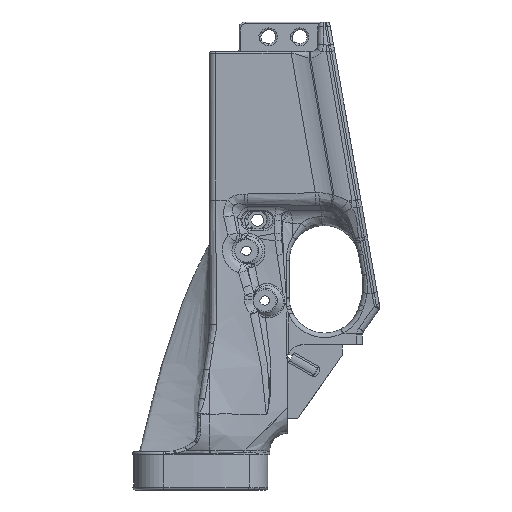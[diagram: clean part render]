
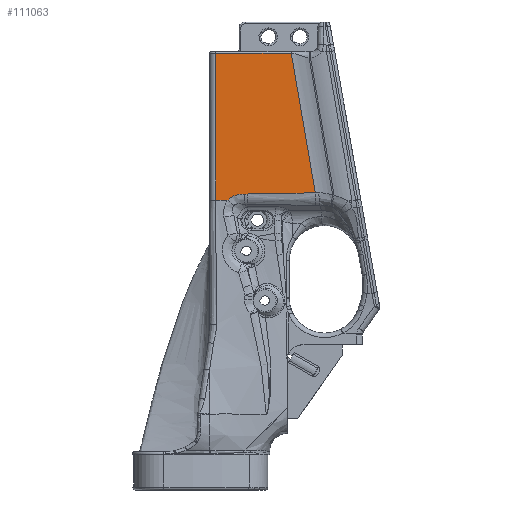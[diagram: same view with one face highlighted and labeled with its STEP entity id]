
A CAD part, left-side view. The second image highlights one B-rep face of the part: STEP entity #111063.
In plain terms, the highlighted planar face has unit normal (-1, 0, 0).
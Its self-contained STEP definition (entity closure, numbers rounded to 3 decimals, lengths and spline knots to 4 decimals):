
#154 = CARTESIAN_POINT ( 'NONE',  ( -0.7, -0.2845, 3.63 ) ) ;
#1696 = EDGE_CURVE ( 'NONE', #95053, #49894, #95486, .T. ) ;
#1853 = CARTESIAN_POINT ( 'NONE',  ( -0.7, -0.2304, 3.63 ) ) ;
#2705 = ORIENTED_EDGE ( 'NONE', *, *, #1696, .T. ) ;
#3995 = CARTESIAN_POINT ( 'NONE',  ( -0.7, -1.7909, 3.7543 ) ) ;
#4014 = DIRECTION ( 'NONE',  ( 0., -1., 0. ) ) ;
#4437 = LINE ( 'NONE', #12462, #68008 ) ;
#8159 = CARTESIAN_POINT ( 'NONE',  ( -0.7, -0.1, 6.12 ) ) ;
#9075 = VECTOR ( 'NONE', #42230, 39.3701 ) ;
#9605 = EDGE_CURVE ( 'NONE', #103485, #88719, #54430, .T. ) ;
#10171 = ORIENTED_EDGE ( 'NONE', *, *, #54507, .F. ) ;
#12462 = CARTESIAN_POINT ( 'NONE',  ( -0.7, 0., 6.12 ) ) ;
#13210 = CARTESIAN_POINT ( 'NONE',  ( -0.7, -0.5916, 3.7336 ) ) ;
#13559 = AXIS2_PLACEMENT_3D ( 'NONE', #17843, #69344, #61894 ) ;
#15915 = CARTESIAN_POINT ( 'NONE',  ( -0.7, -1.4229, 5.8986 ) ) ;
#17333 = EDGE_CURVE ( 'NONE', #108173, #111315, #99951, .T. ) ;
#17843 = CARTESIAN_POINT ( 'NONE',  ( -0.7, -2.8877, 6.15 ) ) ;
#17896 = CARTESIAN_POINT ( 'NONE',  ( -0.7, -0.1, 3.63 ) ) ;
#20760 = EDGE_LOOP ( 'NONE', ( #93236, #26798, #106490, #10171, #74144, #101146, #53672, #2705 ) ) ;
#23035 = CARTESIAN_POINT ( 'NONE',  ( -0.7, -0.4525, 3.7151 ) ) ;
#24162 = CARTESIAN_POINT ( 'NONE',  ( -0.7, -0.3296, 3.6483 ) ) ;
#25581 = CARTESIAN_POINT ( 'NONE',  ( -0.7, -0.3116, 3.63 ) ) ;
#26413 = CARTESIAN_POINT ( 'NONE',  ( -0.7, -0.2304, 3.63 ) ) ;
#26508 = CARTESIAN_POINT ( 'NONE',  ( -0.7, -0.3116, 3.63 ) ) ;
#26798 = ORIENTED_EDGE ( 'NONE', *, *, #48734, .T. ) ;
#28096 = CARTESIAN_POINT ( 'NONE',  ( -0.7, -0.64, 3.7336 ) ) ;
#28221 = CARTESIAN_POINT ( 'NONE',  ( -0.7, -0.1869, 3.63 ) ) ;
#28793 = CARTESIAN_POINT ( 'NONE',  ( -0.7, -0.2304, 3.63 ) ) ;
#29260 = LINE ( 'NONE', #108776, #111168 ) ;
#30536 = CARTESIAN_POINT ( 'NONE',  ( -0.7, -0.3495, 3.6646 ) ) ;
#35581 = FACE_OUTER_BOUND ( 'NONE', #20760, .T. ) ;
#35969 = EDGE_CURVE ( 'NONE', #48324, #95053, #98297, .T. ) ;
#38367 = CARTESIAN_POINT ( 'NONE',  ( -0.7, -1.0236, 3.7336 ) ) ;
#40769 = CARTESIAN_POINT ( 'NONE',  ( -0.7, -0.5916, 3.7336 ) ) ;
#41327 = CARTESIAN_POINT ( 'NONE',  ( -0.7, -0.416, 3.7029 ) ) ;
#42230 = DIRECTION ( 'NONE',  ( 0., 0.169, 0.986 ) ) ;
#47639 = CARTESIAN_POINT ( 'NONE',  ( -0.7, -0.1, 3.63 ) ) ;
#48324 = VERTEX_POINT ( 'NONE', #76389 ) ;
#48734 = EDGE_CURVE ( 'NONE', #110778, #88719, #95185, .T. ) ;
#48803 = CARTESIAN_POINT ( 'NONE',  ( -0.7, -0.3202, 3.6395 ) ) ;
#49894 = VERTEX_POINT ( 'NONE', #61259 ) ;
#53672 = ORIENTED_EDGE ( 'NONE', *, *, #35969, .T. ) ;
#54379 = CARTESIAN_POINT ( 'NONE',  ( -0.7, -1.4073, 3.7543 ) ) ;
#54430 = B_SPLINE_CURVE_WITH_KNOTS ( 'NONE', 3,
 ( #28793, #28221, #62544, #47639 ),
 .UNSPECIFIED., .F., .F.,
 ( 4, 4 ),
 ( 0.64, 0.8438 ),
 .UNSPECIFIED. ) ;
#54507 = EDGE_CURVE ( 'NONE', #108173, #103485, #78418, .T. ) ;
#57945 = CARTESIAN_POINT ( 'NONE',  ( -0.7, -0.5404, 3.732 ) ) ;
#58511 = CARTESIAN_POINT ( 'NONE',  ( -0.7, -0.4899, 3.7243 ) ) ;
#61259 = CARTESIAN_POINT ( 'NONE',  ( -0.7, -1.3849, 6.12 ) ) ;
#61894 = DIRECTION ( 'NONE',  ( 0., 0., 1. ) ) ;
#61949 = CARTESIAN_POINT ( 'NONE',  ( -0.7, -0.1, 5.29 ) ) ;
#62544 = CARTESIAN_POINT ( 'NONE',  ( -0.7, -0.1435, 3.63 ) ) ;
#63112 = CARTESIAN_POINT ( 'NONE',  ( -0.7, -0.2574, 3.63 ) ) ;
#65401 = CARTESIAN_POINT ( 'NONE',  ( -0.7, -0.4649, 3.7186 ) ) ;
#66149 = CARTESIAN_POINT ( 'NONE',  ( -0.7, -0.1, 3.63 ) ) ;
#66530 = CARTESIAN_POINT ( 'NONE',  ( -0.7, -0.3601, 3.6722 ) ) ;
#68008 = VECTOR ( 'NONE', #74804, 39.3701 ) ;
#68396 = EDGE_CURVE ( 'NONE', #49894, #110778, #4437, .T. ) ;
#69344 = DIRECTION ( 'NONE',  ( -1., 0., 0. ) ) ;
#74144 = ORIENTED_EDGE ( 'NONE', *, *, #17333, .T. ) ;
#74534 = CARTESIAN_POINT ( 'NONE',  ( -0.7, -0.5659, 3.7336 ) ) ;
#74737 = EDGE_CURVE ( 'NONE', #111315, #48324, #29260, .T. ) ;
#74804 = DIRECTION ( 'NONE',  ( 0., 1., 0. ) ) ;
#76389 = CARTESIAN_POINT ( 'NONE',  ( -0.7, -0.64, 3.7336 ) ) ;
#78418 = B_SPLINE_CURVE_WITH_KNOTS ( 'NONE', 3,
 ( #26508, #154, #63112, #1853 ),
 .UNSPECIFIED., .F., .F.,
 ( 4, 4 ),
 ( 0.5133, 0.64 ),
 .UNSPECIFIED. ) ;
#79030 = CARTESIAN_POINT ( 'NONE',  ( -0.7, -1.7909, 3.7543 ) ) ;
#87374 = CARTESIAN_POINT ( 'NONE',  ( -0.7, -0.1, 6.12 ) ) ;
#88719 = VERTEX_POINT ( 'NONE', #66149 ) ;
#92869 = CARTESIAN_POINT ( 'NONE',  ( -0.7, -0.3116, 3.63 ) ) ;
#93236 = ORIENTED_EDGE ( 'NONE', *, *, #68396, .T. ) ;
#95053 = VERTEX_POINT ( 'NONE', #79030 ) ;
#95185 = B_SPLINE_CURVE_WITH_KNOTS ( 'NONE', 3,
 ( #8159, #61949, #96312, #17896 ),
 .UNSPECIFIED., .F., .F.,
 ( 4, 4 ),
 ( -0.1525, -0.0893 ),
 .UNSPECIFIED. ) ;
#95486 = LINE ( 'NONE', #15915, #9075 ) ;
#96312 = CARTESIAN_POINT ( 'NONE',  ( -0.7, -0.1, 4.46 ) ) ;
#98297 = B_SPLINE_CURVE_WITH_KNOTS ( 'NONE', 3,
 ( #28096, #38367, #54379, #3995 ),
 .UNSPECIFIED., .F., .F.,
 ( 4, 4 ),
 ( 0.0279, 0.0571 ),
 .UNSPECIFIED. ) ;
#99951 = B_SPLINE_CURVE_WITH_KNOTS ( 'NONE', 3,
 ( #92869, #48803, #24162, #30536, #66530, #100914, #41327, #23035, #65401, #58511, #102014, #57945, #74534, #40769 ),
 .UNSPECIFIED., .F., .F.,
 ( 4, 2, 2, 2, 2, 2, 4 ),
 ( 0., 0.001, 0.002, 0.0039, 0.0049, 0.0059, 0.0078 ),
 .UNSPECIFIED. ) ;
#100914 = CARTESIAN_POINT ( 'NONE',  ( -0.7, -0.3928, 3.6924 ) ) ;
#101146 = ORIENTED_EDGE ( 'NONE', *, *, #74737, .T. ) ;
#102014 = CARTESIAN_POINT ( 'NONE',  ( -0.7, -0.5025, 3.7266 ) ) ;
#103161 = PLANE ( 'NONE',  #13559 ) ;
#103485 = VERTEX_POINT ( 'NONE', #26413 ) ;
#106490 = ORIENTED_EDGE ( 'NONE', *, *, #9605, .F. ) ;
#108173 = VERTEX_POINT ( 'NONE', #25581 ) ;
#108776 = CARTESIAN_POINT ( 'NONE',  ( -0.7, -2.8877, 3.7336 ) ) ;
#110778 = VERTEX_POINT ( 'NONE', #87374 ) ;
#111063 = ADVANCED_FACE ( 'NONE', ( #35581 ), #103161, .T. ) ;
#111168 = VECTOR ( 'NONE', #4014, 39.3701 ) ;
#111315 = VERTEX_POINT ( 'NONE', #13210 ) ;
